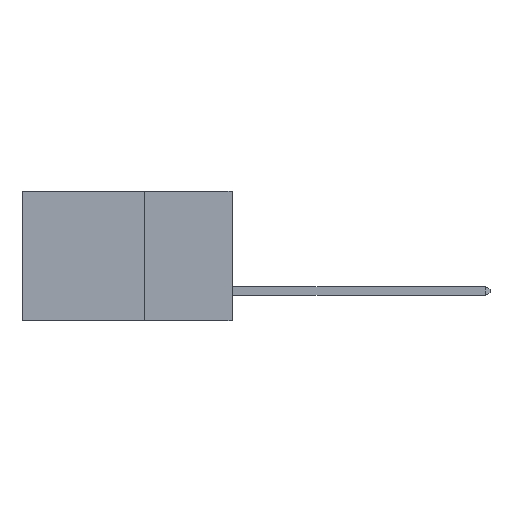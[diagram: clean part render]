
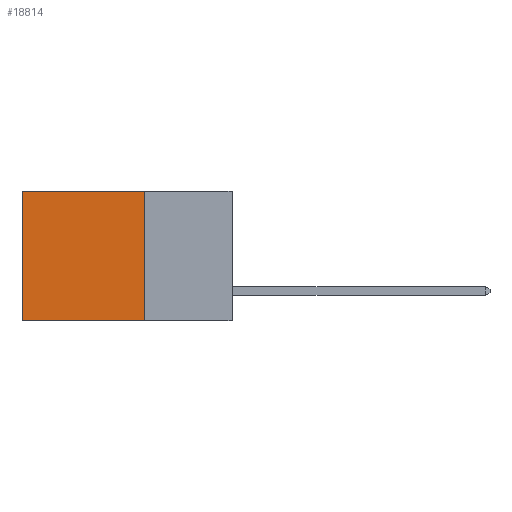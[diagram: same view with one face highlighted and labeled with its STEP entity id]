
A CAD part, left-side view. The second image highlights one B-rep face of the part: STEP entity #18814.
In plain terms, the highlighted planar face has unit normal (-1, 0, 0).
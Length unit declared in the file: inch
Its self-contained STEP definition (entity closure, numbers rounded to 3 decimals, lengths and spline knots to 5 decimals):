
#253 = VECTOR ( 'NONE', #21677, 39.37008 ) ;
#488 = VERTEX_POINT ( 'NONE', #12605 ) ;
#1486 = ORIENTED_EDGE ( 'NONE', *, *, #19889, .T. ) ;
#2010 = CARTESIAN_POINT ( 'NONE',  ( 0.2875, 0.25, -0.37 ) ) ;
#2652 = LINE ( 'NONE', #2010, #17814 ) ;
#2847 = VERTEX_POINT ( 'NONE', #11457 ) ;
#4050 = DIRECTION ( 'NONE',  ( 0., 1., 0. ) ) ;
#6401 = VERTEX_POINT ( 'NONE', #8608 ) ;
#6501 = CARTESIAN_POINT ( 'NONE',  ( 0.2875, 0.25, 0. ) ) ;
#6831 = DIRECTION ( 'NONE',  ( 0., 0., -1. ) ) ;
#7216 = ORIENTED_EDGE ( 'NONE', *, *, #19742, .F. ) ;
#7724 = CARTESIAN_POINT ( 'NONE',  ( 0.2875, 0.25, 0. ) ) ;
#8439 = DIRECTION ( 'NONE',  ( 0., 0., -1. ) ) ;
#8608 = CARTESIAN_POINT ( 'NONE',  ( 0.2875, 0.25, -0.37 ) ) ;
#9082 = ORIENTED_EDGE ( 'NONE', *, *, #18971, .T. ) ;
#9951 = CARTESIAN_POINT ( 'NONE',  ( 0.2875, 0.25, 0. ) ) ;
#10759 = CARTESIAN_POINT ( 'NONE',  ( 0.2875, 0.6, 0. ) ) ;
#11060 = DIRECTION ( 'NONE',  ( 1., 0., 0. ) ) ;
#11457 = CARTESIAN_POINT ( 'NONE',  ( 0.2875, 0.6, -0.37 ) ) ;
#12605 = CARTESIAN_POINT ( 'NONE',  ( 0.2875, 0.6, 0. ) ) ;
#13254 = FACE_OUTER_BOUND ( 'NONE', #15880, .T. ) ;
#13885 = EDGE_CURVE ( 'NONE', #6401, #2847, #2652, .T. ) ;
#14811 = LINE ( 'NONE', #9951, #253 ) ;
#15880 = EDGE_LOOP ( 'NONE', ( #1486, #18741, #7216, #9082 ) ) ;
#16177 = AXIS2_PLACEMENT_3D ( 'NONE', #20834, #11060, #24677 ) ;
#16648 = VECTOR ( 'NONE', #8439, 39.37008 ) ;
#16654 = VERTEX_POINT ( 'NONE', #7724 ) ;
#17814 = VECTOR ( 'NONE', #4050, 39.37008 ) ;
#17882 = LINE ( 'NONE', #6501, #16648 ) ;
#18741 = ORIENTED_EDGE ( 'NONE', *, *, #13885, .F. ) ;
#18774 = LINE ( 'NONE', #10759, #23859 ) ;
#18814 = ADVANCED_FACE ( 'NONE', ( #13254 ), #22759, .F. ) ;
#18971 = EDGE_CURVE ( 'NONE', #16654, #488, #14811, .T. ) ;
#19742 = EDGE_CURVE ( 'NONE', #16654, #6401, #17882, .T. ) ;
#19889 = EDGE_CURVE ( 'NONE', #488, #2847, #18774, .T. ) ;
#20834 = CARTESIAN_POINT ( 'NONE',  ( 0.2875, 0.25, 0. ) ) ;
#21677 = DIRECTION ( 'NONE',  ( 0., 1., 0. ) ) ;
#22759 = PLANE ( 'NONE',  #16177 ) ;
#23859 = VECTOR ( 'NONE', #6831, 39.37008 ) ;
#24677 = DIRECTION ( 'NONE',  ( 0., 0., -1. ) ) ;
